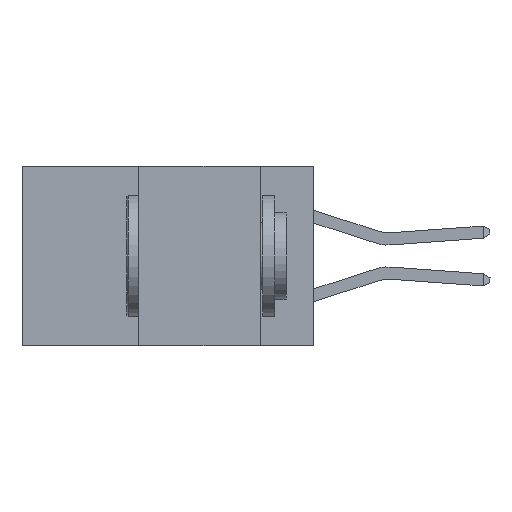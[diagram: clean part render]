
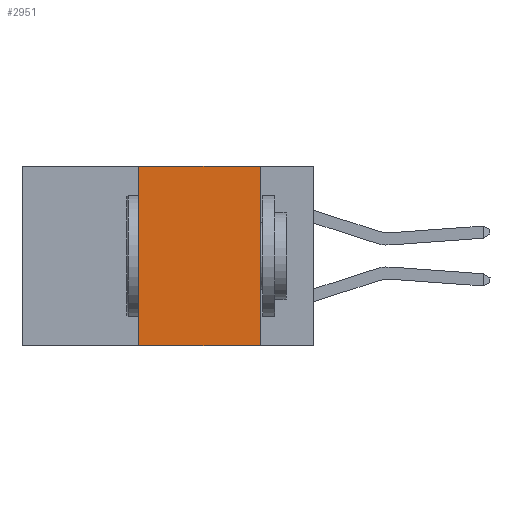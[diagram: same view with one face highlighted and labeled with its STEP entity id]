
A CAD part, left-side view. The second image highlights one B-rep face of the part: STEP entity #2951.
In plain terms, the highlighted planar face has unit normal (-1, 0, 0).
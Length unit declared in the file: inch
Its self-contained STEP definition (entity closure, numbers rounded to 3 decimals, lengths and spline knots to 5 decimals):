
#677 = ORIENTED_EDGE ( 'NONE', *, *, #3202, .F. ) ;
#730 = CARTESIAN_POINT ( 'NONE',  ( 0., 0.11, 0. ) ) ;
#1035 = CARTESIAN_POINT ( 'NONE',  ( 0., 0.36, 0. ) ) ;
#1794 = VECTOR ( 'NONE', #29027, 39.37008 ) ;
#2265 = VERTEX_POINT ( 'NONE', #5506 ) ;
#2951 = ADVANCED_FACE ( 'NONE', ( #4852 ), #27336, .F. ) ;
#3127 = ORIENTED_EDGE ( 'NONE', *, *, #12550, .F. ) ;
#3202 = EDGE_CURVE ( 'NONE', #2265, #22751, #13891, .T. ) ;
#4537 = DIRECTION ( 'NONE',  ( 1., 0., 0. ) ) ;
#4852 = FACE_OUTER_BOUND ( 'NONE', #12916, .T. ) ;
#5506 = CARTESIAN_POINT ( 'NONE',  ( 0., 0.36, -0.37 ) ) ;
#8290 = DIRECTION ( 'NONE',  ( 0., 0., -1. ) ) ;
#8524 = LINE ( 'NONE', #26487, #1794 ) ;
#9346 = LINE ( 'NONE', #26763, #28510 ) ;
#9631 = CARTESIAN_POINT ( 'NONE',  ( 0., 0.11, -0.37 ) ) ;
#12035 = DIRECTION ( 'NONE',  ( 0., 0., -1. ) ) ;
#12156 = EDGE_CURVE ( 'NONE', #2265, #27578, #8524, .T. ) ;
#12550 = EDGE_CURVE ( 'NONE', #22091, #27578, #20670, .T. ) ;
#12916 = EDGE_LOOP ( 'NONE', ( #3127, #31798, #677, #18434 ) ) ;
#13891 = LINE ( 'NONE', #24699, #24053 ) ;
#14984 = DIRECTION ( 'NONE',  ( 0., 0., 1. ) ) ;
#16481 = CARTESIAN_POINT ( 'NONE',  ( 0., 0.11, 0. ) ) ;
#18434 = ORIENTED_EDGE ( 'NONE', *, *, #12156, .T. ) ;
#20670 = LINE ( 'NONE', #730, #22617 ) ;
#22091 = VERTEX_POINT ( 'NONE', #16481 ) ;
#22207 = CARTESIAN_POINT ( 'NONE',  ( 0., 0.6, 0. ) ) ;
#22617 = VECTOR ( 'NONE', #8290, 39.37008 ) ;
#22751 = VERTEX_POINT ( 'NONE', #1035 ) ;
#22799 = AXIS2_PLACEMENT_3D ( 'NONE', #22207, #4537, #12035 ) ;
#24053 = VECTOR ( 'NONE', #14984, 39.37008 ) ;
#24149 = DIRECTION ( 'NONE',  ( 0., -1., 0. ) ) ;
#24699 = CARTESIAN_POINT ( 'NONE',  ( 0., 0.36, 0. ) ) ;
#25362 = EDGE_CURVE ( 'NONE', #22751, #22091, #9346, .T. ) ;
#26487 = CARTESIAN_POINT ( 'NONE',  ( 0., 0.6, -0.37 ) ) ;
#26763 = CARTESIAN_POINT ( 'NONE',  ( 0., 0.6, 0. ) ) ;
#27336 = PLANE ( 'NONE',  #22799 ) ;
#27578 = VERTEX_POINT ( 'NONE', #9631 ) ;
#28510 = VECTOR ( 'NONE', #24149, 39.37008 ) ;
#29027 = DIRECTION ( 'NONE',  ( 0., -1., 0. ) ) ;
#31798 = ORIENTED_EDGE ( 'NONE', *, *, #25362, .F. ) ;
